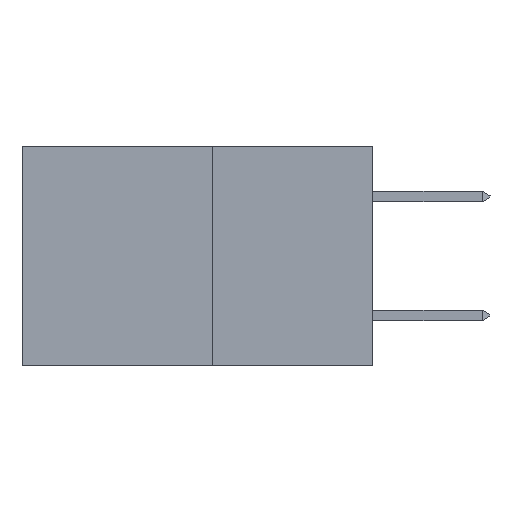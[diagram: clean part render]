
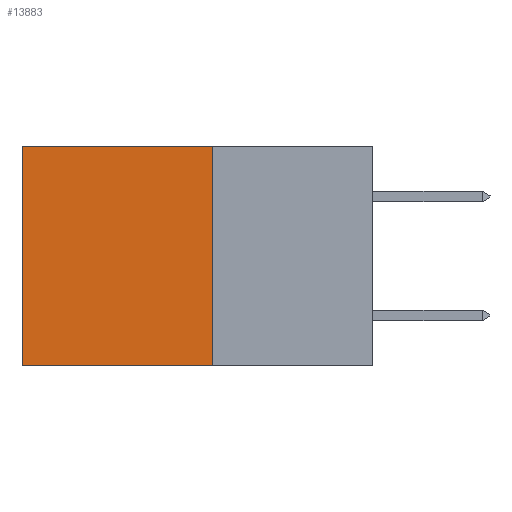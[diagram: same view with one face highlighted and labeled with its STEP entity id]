
A CAD part, left-side view. The second image highlights one B-rep face of the part: STEP entity #13883.
In plain terms, the highlighted planar face has unit normal (-1, 0, 0).
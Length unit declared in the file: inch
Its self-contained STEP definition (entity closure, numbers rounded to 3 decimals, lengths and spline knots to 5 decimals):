
#352 = VERTEX_POINT ( 'NONE', #19327 ) ;
#364 = FACE_OUTER_BOUND ( 'NONE', #8092, .T. ) ;
#524 = ORIENTED_EDGE ( 'NONE', *, *, #12584, .F. ) ;
#741 = DIRECTION ( 'NONE',  ( 0., 0., -1. ) ) ;
#1518 = CARTESIAN_POINT ( 'NONE',  ( 0.277, 0.27, -0.37 ) ) ;
#2983 = ORIENTED_EDGE ( 'NONE', *, *, #5408, .F. ) ;
#4380 = CARTESIAN_POINT ( 'NONE',  ( 0.277, 0.27, -0.37 ) ) ;
#5054 = LINE ( 'NONE', #1518, #16853 ) ;
#5408 = EDGE_CURVE ( 'NONE', #23591, #352, #5054, .T. ) ;
#5982 = CARTESIAN_POINT ( 'NONE',  ( 0.277, 0.59, -0.37 ) ) ;
#6603 = DIRECTION ( 'NONE',  ( 0., 0., -1. ) ) ;
#7339 = ORIENTED_EDGE ( 'NONE', *, *, #12974, .T. ) ;
#8092 = EDGE_LOOP ( 'NONE', ( #7339, #524, #2983, #15886 ) ) ;
#8225 = DIRECTION ( 'NONE',  ( 0., 0., -1. ) ) ;
#10111 = VECTOR ( 'NONE', #26873, 39.37008 ) ;
#10141 = LINE ( 'NONE', #20667, #27137 ) ;
#12165 = EDGE_CURVE ( 'NONE', #23591, #22290, #10141, .T. ) ;
#12584 = EDGE_CURVE ( 'NONE', #352, #16001, #16022, .T. ) ;
#12974 = EDGE_CURVE ( 'NONE', #22290, #16001, #23661, .T. ) ;
#13587 = CARTESIAN_POINT ( 'NONE',  ( 0.277, 0.27, -0.37 ) ) ;
#13883 = ADVANCED_FACE ( 'NONE', ( #364 ), #24269, .F. ) ;
#14106 = CARTESIAN_POINT ( 'NONE',  ( 0.277, 0.59, 0. ) ) ;
#15886 = ORIENTED_EDGE ( 'NONE', *, *, #12165, .T. ) ;
#16001 = VERTEX_POINT ( 'NONE', #17632 ) ;
#16022 = LINE ( 'NONE', #13587, #10111 ) ;
#16853 = VECTOR ( 'NONE', #741, 39.37008 ) ;
#17632 = CARTESIAN_POINT ( 'NONE',  ( 0.277, 0.59, -0.37 ) ) ;
#17767 = VECTOR ( 'NONE', #8225, 39.37008 ) ;
#19285 = AXIS2_PLACEMENT_3D ( 'NONE', #4380, #19898, #6603 ) ;
#19327 = CARTESIAN_POINT ( 'NONE',  ( 0.277, 0.27, -0.37 ) ) ;
#19898 = DIRECTION ( 'NONE',  ( 1., 0., 0. ) ) ;
#20667 = CARTESIAN_POINT ( 'NONE',  ( 0.277, 0.27, 0. ) ) ;
#20918 = CARTESIAN_POINT ( 'NONE',  ( 0.277, 0.27, 0. ) ) ;
#22290 = VERTEX_POINT ( 'NONE', #14106 ) ;
#22909 = DIRECTION ( 'NONE',  ( 0., 1., 0. ) ) ;
#23591 = VERTEX_POINT ( 'NONE', #20918 ) ;
#23661 = LINE ( 'NONE', #5982, #17767 ) ;
#24269 = PLANE ( 'NONE',  #19285 ) ;
#26873 = DIRECTION ( 'NONE',  ( 0., 1., 0. ) ) ;
#27137 = VECTOR ( 'NONE', #22909, 39.37008 ) ;
